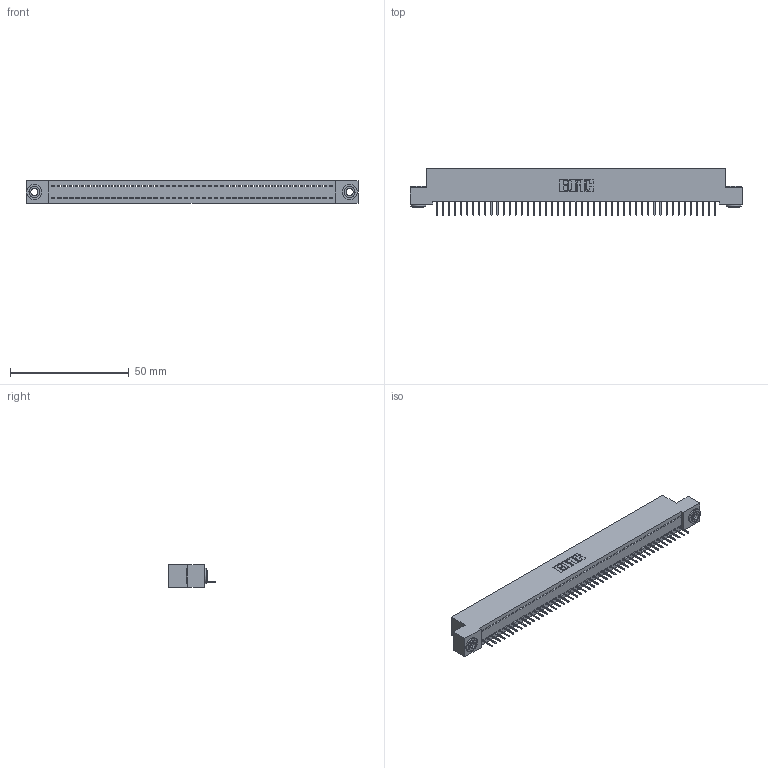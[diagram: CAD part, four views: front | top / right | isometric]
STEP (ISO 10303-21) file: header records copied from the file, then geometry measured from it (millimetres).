
FILE_DESCRIPTION (( 'STEP AP203' ), '1' );
FILE_NAME ('342-047-524-103.STEP', '2018-08-12T17:02:01', ( '' ), ( '' ), 'SwSTEP 2.0', 'SolidWorks 2016', '' );
FILE_SCHEMA (( 'CONFIG_CONTROL_DESIGN' ));
Length unit declared in the file: inch
Products named in the file (4): 342 Part_.156 TH; 345-292-001_345-293-124; 342-250-002_345-250-002-102; 342-047-524-103
Assembly tree (50 placements, depth 2):
  342-047-524-103
    342 Part_.156 TH
    345-292-001_345-293-124  x47
    342-250-002_345-250-002-102  x2
Bounding box: 139.7 x 19.69 x 9.4 mm (x, y, z)
Volume: 12104.5 mm3; surface area: 17517.7 mm2
Topology: 50 solids, 50 shells, 3062 faces, 8835 edges, 5698 vertices
Faces by surface type: plane 2332, cylinder 722, cone 8
Entity records: 28678 total; most frequent: CARTESIAN_POINT 4922, ORIENTED_EDGE 4898, DIRECTION 4177, EDGE_CURVE 2449, VECTOR 2301, LINE 2301, VERTEX_POINT 1626, AXIS2_PLACEMENT_3D 938
